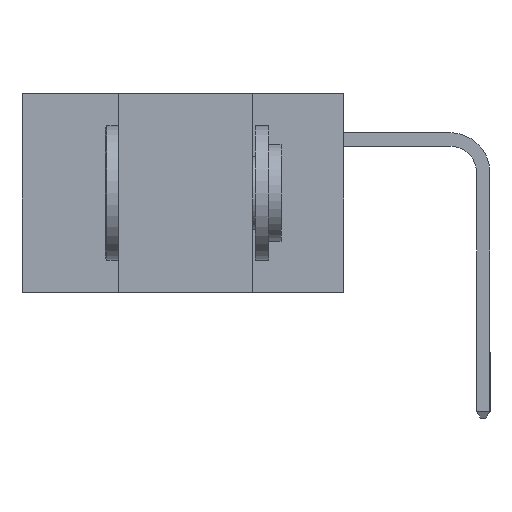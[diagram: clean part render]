
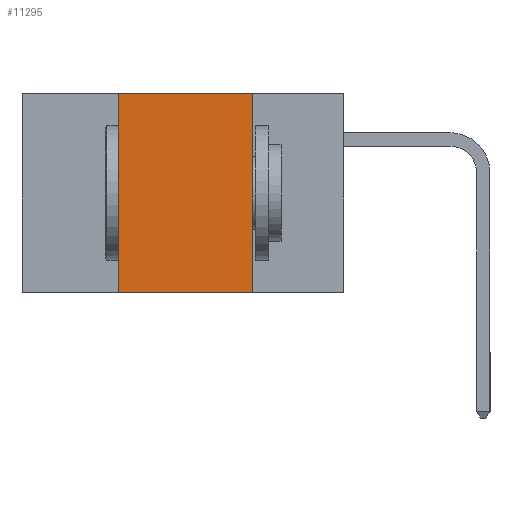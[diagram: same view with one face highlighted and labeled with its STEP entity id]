
A CAD part, left-side view. The second image highlights one B-rep face of the part: STEP entity #11295.
In plain terms, the highlighted planar face has unit normal (-1, 0, 0).
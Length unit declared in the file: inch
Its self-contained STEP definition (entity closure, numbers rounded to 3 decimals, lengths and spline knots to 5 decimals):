
#1129 = EDGE_CURVE ( 'NONE', #15044, #15946, #12903, .T. ) ;
#1599 = CARTESIAN_POINT ( 'NONE',  ( 0., 0.6, -0.37 ) ) ;
#1815 = CARTESIAN_POINT ( 'NONE',  ( 0., 0.42, -0.37 ) ) ;
#2777 = VERTEX_POINT ( 'NONE', #11306 ) ;
#3435 = CARTESIAN_POINT ( 'NONE',  ( 0., 0.6, 0. ) ) ;
#4464 = FACE_OUTER_BOUND ( 'NONE', #19484, .T. ) ;
#4554 = DIRECTION ( 'NONE',  ( 1., 0., 0. ) ) ;
#4622 = LINE ( 'NONE', #3435, #4707 ) ;
#4707 = VECTOR ( 'NONE', #11079, 39.37008 ) ;
#5561 = CARTESIAN_POINT ( 'NONE',  ( 0., 0.17, -0.37 ) ) ;
#5570 = VECTOR ( 'NONE', #14666, 39.37008 ) ;
#5782 = AXIS2_PLACEMENT_3D ( 'NONE', #15213, #4554, #19926 ) ;
#6029 = VECTOR ( 'NONE', #18572, 39.37008 ) ;
#6557 = ORIENTED_EDGE ( 'NONE', *, *, #17144, .F. ) ;
#7708 = ORIENTED_EDGE ( 'NONE', *, *, #1129, .T. ) ;
#8031 = DIRECTION ( 'NONE',  ( 0., -1., 0. ) ) ;
#9786 = VECTOR ( 'NONE', #8031, 39.37008 ) ;
#10300 = CARTESIAN_POINT ( 'NONE',  ( 0., 0.42, -0.37 ) ) ;
#11079 = DIRECTION ( 'NONE',  ( 0., -1., 0. ) ) ;
#11295 = ADVANCED_FACE ( 'NONE', ( #4464 ), #18963, .F. ) ;
#11306 = CARTESIAN_POINT ( 'NONE',  ( 0., 0.42, 0. ) ) ;
#11602 = ORIENTED_EDGE ( 'NONE', *, *, #13687, .F. ) ;
#12201 = CARTESIAN_POINT ( 'NONE',  ( 0., 0.17, -0.37 ) ) ;
#12355 = VERTEX_POINT ( 'NONE', #15644 ) ;
#12903 = LINE ( 'NONE', #1599, #9786 ) ;
#13687 = EDGE_CURVE ( 'NONE', #15044, #2777, #14574, .T. ) ;
#14574 = LINE ( 'NONE', #1815, #5570 ) ;
#14666 = DIRECTION ( 'NONE',  ( 0., 0., 1. ) ) ;
#15044 = VERTEX_POINT ( 'NONE', #10300 ) ;
#15213 = CARTESIAN_POINT ( 'NONE',  ( 0., 0.6, 0. ) ) ;
#15607 = ORIENTED_EDGE ( 'NONE', *, *, #17811, .F. ) ;
#15644 = CARTESIAN_POINT ( 'NONE',  ( 0., 0.17, 0. ) ) ;
#15946 = VERTEX_POINT ( 'NONE', #5561 ) ;
#16873 = LINE ( 'NONE', #12201, #6029 ) ;
#17144 = EDGE_CURVE ( 'NONE', #12355, #15946, #16873, .T. ) ;
#17811 = EDGE_CURVE ( 'NONE', #2777, #12355, #4622, .T. ) ;
#18572 = DIRECTION ( 'NONE',  ( 0., 0., -1. ) ) ;
#18963 = PLANE ( 'NONE',  #5782 ) ;
#19484 = EDGE_LOOP ( 'NONE', ( #6557, #15607, #11602, #7708 ) ) ;
#19926 = DIRECTION ( 'NONE',  ( 0., 0., -1. ) ) ;
